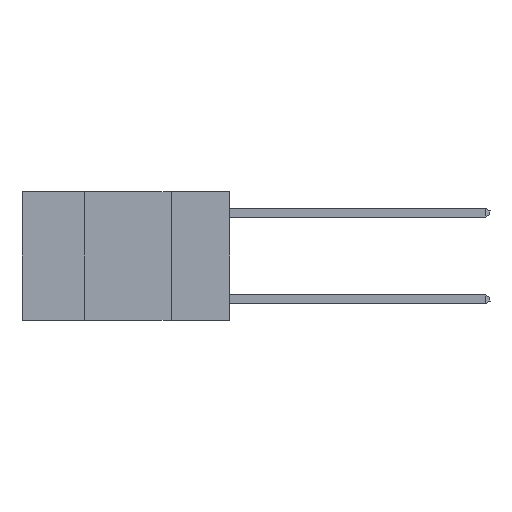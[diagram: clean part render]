
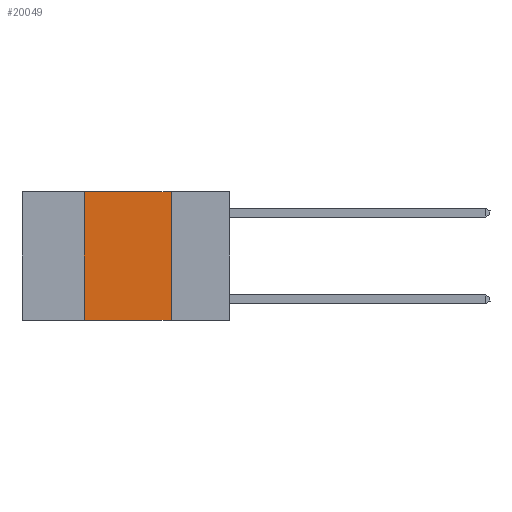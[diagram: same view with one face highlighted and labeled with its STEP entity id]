
A CAD part, left-side view. The second image highlights one B-rep face of the part: STEP entity #20049.
In plain terms, the highlighted planar face has unit normal (-1, 0, 0).
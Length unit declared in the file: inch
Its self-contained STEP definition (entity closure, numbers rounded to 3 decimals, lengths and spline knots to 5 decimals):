
#91 = FACE_OUTER_BOUND ( 'NONE', #19313, .T. ) ;
#554 = LINE ( 'NONE', #9170, #12763 ) ;
#908 = DIRECTION ( 'NONE',  ( 0., -1., 0. ) ) ;
#1737 = LINE ( 'NONE', #8969, #14956 ) ;
#2267 = AXIS2_PLACEMENT_3D ( 'NONE', #4133, #8901, #19948 ) ;
#3058 = VERTEX_POINT ( 'NONE', #10003 ) ;
#3446 = VECTOR ( 'NONE', #908, 39.37008 ) ;
#4133 = CARTESIAN_POINT ( 'NONE',  ( 0., 0.6, 0. ) ) ;
#5326 = EDGE_CURVE ( 'NONE', #16841, #8189, #554, .T. ) ;
#6276 = CARTESIAN_POINT ( 'NONE',  ( 0., 0.42, -0.37 ) ) ;
#7288 = VERTEX_POINT ( 'NONE', #8548 ) ;
#7443 = EDGE_CURVE ( 'NONE', #7288, #3058, #1737, .T. ) ;
#7535 = CARTESIAN_POINT ( 'NONE',  ( 0., 0.42, 0. ) ) ;
#8189 = VERTEX_POINT ( 'NONE', #7535 ) ;
#8548 = CARTESIAN_POINT ( 'NONE',  ( 0., 0.17, 0. ) ) ;
#8901 = DIRECTION ( 'NONE',  ( 1., 0., 0. ) ) ;
#8969 = CARTESIAN_POINT ( 'NONE',  ( 0., 0.17, 0. ) ) ;
#9170 = CARTESIAN_POINT ( 'NONE',  ( 0., 0.42, 0. ) ) ;
#10003 = CARTESIAN_POINT ( 'NONE',  ( 0., 0.17, -0.37 ) ) ;
#10048 = ORIENTED_EDGE ( 'NONE', *, *, #7443, .F. ) ;
#11584 = LINE ( 'NONE', #17287, #15807 ) ;
#12763 = VECTOR ( 'NONE', #20225, 39.37008 ) ;
#14140 = DIRECTION ( 'NONE',  ( 0., -1., 0. ) ) ;
#14297 = EDGE_CURVE ( 'NONE', #16841, #3058, #19773, .T. ) ;
#14551 = ORIENTED_EDGE ( 'NONE', *, *, #18892, .F. ) ;
#14956 = VECTOR ( 'NONE', #20020, 39.37008 ) ;
#15533 = ORIENTED_EDGE ( 'NONE', *, *, #5326, .F. ) ;
#15807 = VECTOR ( 'NONE', #14140, 39.37008 ) ;
#16841 = VERTEX_POINT ( 'NONE', #6276 ) ;
#17287 = CARTESIAN_POINT ( 'NONE',  ( 0., 0.6, 0. ) ) ;
#18892 = EDGE_CURVE ( 'NONE', #8189, #7288, #11584, .T. ) ;
#19313 = EDGE_LOOP ( 'NONE', ( #10048, #14551, #15533, #20361 ) ) ;
#19773 = LINE ( 'NONE', #19865, #3446 ) ;
#19865 = CARTESIAN_POINT ( 'NONE',  ( 0., 0.6, -0.37 ) ) ;
#19884 = PLANE ( 'NONE',  #2267 ) ;
#19948 = DIRECTION ( 'NONE',  ( 0., 0., -1. ) ) ;
#20020 = DIRECTION ( 'NONE',  ( 0., 0., -1. ) ) ;
#20049 = ADVANCED_FACE ( 'NONE', ( #91 ), #19884, .F. ) ;
#20225 = DIRECTION ( 'NONE',  ( 0., 0., 1. ) ) ;
#20361 = ORIENTED_EDGE ( 'NONE', *, *, #14297, .T. ) ;
